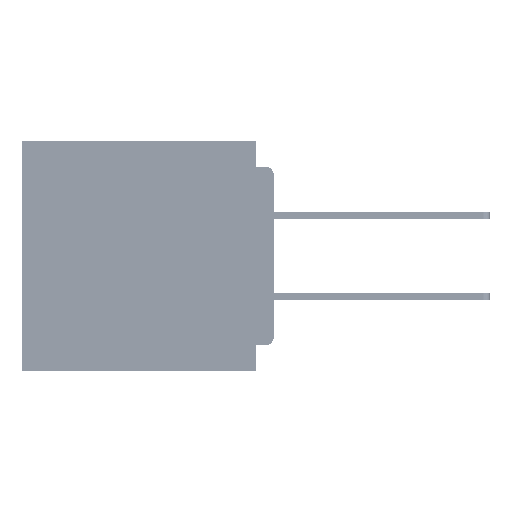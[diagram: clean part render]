
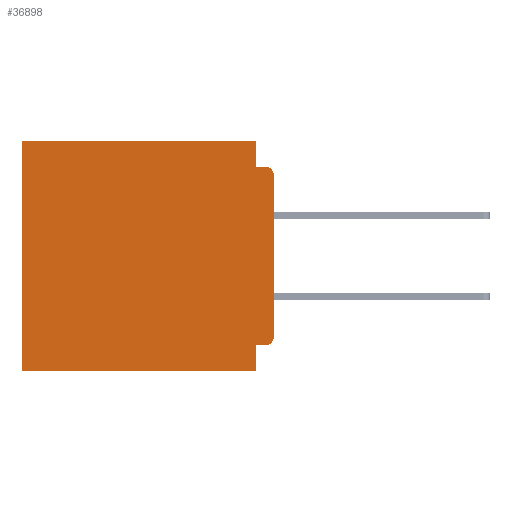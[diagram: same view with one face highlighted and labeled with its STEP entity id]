
A CAD part, left-side view. The second image highlights one B-rep face of the part: STEP entity #36898.
In plain terms, the highlighted planar face has unit normal (-1, 0, 0).
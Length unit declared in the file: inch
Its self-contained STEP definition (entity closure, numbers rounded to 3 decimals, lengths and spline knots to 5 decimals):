
#487 = VECTOR ( 'NONE', #36995, 39.37008 ) ;
#826 = DIRECTION ( 'NONE',  ( 0., -1., 0. ) ) ;
#1412 = EDGE_CURVE ( 'NONE', #47706, #27808, #40963, .T. ) ;
#2848 = DIRECTION ( 'NONE',  ( 0., 0., -1. ) ) ;
#3348 = ORIENTED_EDGE ( 'NONE', *, *, #37753, .F. ) ;
#4889 = VECTOR ( 'NONE', #64248, 39.37008 ) ;
#5545 = ORIENTED_EDGE ( 'NONE', *, *, #58320, .F. ) ;
#6227 = VECTOR ( 'NONE', #2848, 39.37008 ) ;
#6759 = CARTESIAN_POINT ( 'NONE',  ( 0.3, 0.031, -0.045 ) ) ;
#8298 = VERTEX_POINT ( 'NONE', #59583 ) ;
#8503 = LINE ( 'NONE', #52040, #49898 ) ;
#9433 = DIRECTION ( 'NONE',  ( 0., 0., -1. ) ) ;
#9648 = VECTOR ( 'NONE', #52516, 39.37008 ) ;
#11014 = EDGE_CURVE ( 'NONE', #61028, #56909, #8503, .T. ) ;
#11951 = CARTESIAN_POINT ( 'NONE',  ( 0.3, 0.015, -0.355 ) ) ;
#12437 = DIRECTION ( 'NONE',  ( 0., 0., -1. ) ) ;
#12934 = VERTEX_POINT ( 'NONE', #11951 ) ;
#19349 = CARTESIAN_POINT ( 'NONE',  ( 0.3, 0., -0.06 ) ) ;
#19749 = ORIENTED_EDGE ( 'NONE', *, *, #46625, .T. ) ;
#19824 = ORIENTED_EDGE ( 'NONE', *, *, #23410, .F. ) ;
#19858 = EDGE_CURVE ( 'NONE', #12934, #68266, #35274, .T. ) ;
#20147 = CARTESIAN_POINT ( 'NONE',  ( 0.3, 0., -0.4 ) ) ;
#20202 = DIRECTION ( 'NONE',  ( -1., 0., 0. ) ) ;
#20406 = DIRECTION ( 'NONE',  ( -1., 0., 0. ) ) ;
#21000 = EDGE_CURVE ( 'NONE', #47706, #51562, #29183, .T. ) ;
#22382 = LINE ( 'NONE', #28746, #41350 ) ;
#23410 = EDGE_CURVE ( 'NONE', #8298, #57819, #52736, .T. ) ;
#24838 = CARTESIAN_POINT ( 'NONE',  ( 0.3, 0.031, -0.4 ) ) ;
#25645 = CARTESIAN_POINT ( 'NONE',  ( 0.3, 0., -0.34 ) ) ;
#26329 = EDGE_CURVE ( 'NONE', #68266, #8298, #34617, .T. ) ;
#26506 = CARTESIAN_POINT ( 'NONE',  ( 0.3, 0., -0.355 ) ) ;
#27311 = ORIENTED_EDGE ( 'NONE', *, *, #19858, .F. ) ;
#27808 = VERTEX_POINT ( 'NONE', #51575 ) ;
#28276 = ORIENTED_EDGE ( 'NONE', *, *, #26329, .F. ) ;
#28746 = CARTESIAN_POINT ( 'NONE',  ( 0.3, 0.437, -0.4 ) ) ;
#29183 = LINE ( 'NONE', #58269, #487 ) ;
#30254 = DIRECTION ( 'NONE',  ( 0., 0., -1. ) ) ;
#30888 = PLANE ( 'NONE',  #50365 ) ;
#34617 = LINE ( 'NONE', #24838, #61672 ) ;
#35274 = LINE ( 'NONE', #26506, #4889 ) ;
#36310 = CARTESIAN_POINT ( 'NONE',  ( 0.3, 0., -0.4 ) ) ;
#36898 = ADVANCED_FACE ( 'NONE', ( #60589 ), #30888, .F. ) ;
#36995 = DIRECTION ( 'NONE',  ( 0., 0., -1. ) ) ;
#37696 = AXIS2_PLACEMENT_3D ( 'NONE', #52792, #20406, #58209 ) ;
#37753 = EDGE_CURVE ( 'NONE', #46304, #27808, #37769, .T. ) ;
#37769 = LINE ( 'NONE', #38598, #64764 ) ;
#38598 = CARTESIAN_POINT ( 'NONE',  ( 0.3, 0., -0.045 ) ) ;
#40812 = ORIENTED_EDGE ( 'NONE', *, *, #21000, .F. ) ;
#40963 = CIRCLE ( 'NONE', #52365, 0.015 ) ;
#41159 = ORIENTED_EDGE ( 'NONE', *, *, #1412, .T. ) ;
#41350 = VECTOR ( 'NONE', #12437, 39.37008 ) ;
#41779 = DIRECTION ( 'NONE',  ( 1., 0., 0. ) ) ;
#43084 = ORIENTED_EDGE ( 'NONE', *, *, #60879, .T. ) ;
#46196 = CARTESIAN_POINT ( 'NONE',  ( 0.3, 0.031, 0. ) ) ;
#46304 = VERTEX_POINT ( 'NONE', #6759 ) ;
#46625 = EDGE_CURVE ( 'NONE', #12934, #51562, #54628, .T. ) ;
#47706 = VERTEX_POINT ( 'NONE', #19349 ) ;
#49898 = VECTOR ( 'NONE', #57455, 39.37008 ) ;
#50365 = AXIS2_PLACEMENT_3D ( 'NONE', #36310, #41779, #9433 ) ;
#50807 = EDGE_LOOP ( 'NONE', ( #40812, #41159, #3348, #5545, #69065, #43084, #19824, #28276, #27311, #19749 ) ) ;
#51051 = LINE ( 'NONE', #56892, #6227 ) ;
#51562 = VERTEX_POINT ( 'NONE', #25645 ) ;
#51575 = CARTESIAN_POINT ( 'NONE',  ( 0.3, 0.015, -0.045 ) ) ;
#52040 = CARTESIAN_POINT ( 'NONE',  ( 0.3, 0., 0. ) ) ;
#52365 = AXIS2_PLACEMENT_3D ( 'NONE', #52585, #20202, #58007 ) ;
#52516 = DIRECTION ( 'NONE',  ( 0., 1., 0. ) ) ;
#52585 = CARTESIAN_POINT ( 'NONE',  ( 0.3, 0.015, -0.06 ) ) ;
#52736 = LINE ( 'NONE', #20147, #9648 ) ;
#52792 = CARTESIAN_POINT ( 'NONE',  ( 0.3, 0.015, -0.34 ) ) ;
#54628 = CIRCLE ( 'NONE', #37696, 0.015 ) ;
#54936 = CARTESIAN_POINT ( 'NONE',  ( 0.3, 0.437, 0. ) ) ;
#56892 = CARTESIAN_POINT ( 'NONE',  ( 0.3, 0.031, 0. ) ) ;
#56909 = VERTEX_POINT ( 'NONE', #54936 ) ;
#57455 = DIRECTION ( 'NONE',  ( 0., 1., 0. ) ) ;
#57819 = VERTEX_POINT ( 'NONE', #58160 ) ;
#58007 = DIRECTION ( 'NONE',  ( 0., 0., -1. ) ) ;
#58160 = CARTESIAN_POINT ( 'NONE',  ( 0.3, 0.437, -0.4 ) ) ;
#58209 = DIRECTION ( 'NONE',  ( 0., 0., -1. ) ) ;
#58269 = CARTESIAN_POINT ( 'NONE',  ( 0.3, 0., -0.4 ) ) ;
#58320 = EDGE_CURVE ( 'NONE', #61028, #46304, #51051, .T. ) ;
#59583 = CARTESIAN_POINT ( 'NONE',  ( 0.3, 0.031, -0.4 ) ) ;
#60589 = FACE_OUTER_BOUND ( 'NONE', #50807, .T. ) ;
#60879 = EDGE_CURVE ( 'NONE', #56909, #57819, #22382, .T. ) ;
#61028 = VERTEX_POINT ( 'NONE', #46196 ) ;
#61672 = VECTOR ( 'NONE', #30254, 39.37008 ) ;
#61834 = CARTESIAN_POINT ( 'NONE',  ( 0.3, 0.031, -0.355 ) ) ;
#64248 = DIRECTION ( 'NONE',  ( 0., 1., 0. ) ) ;
#64764 = VECTOR ( 'NONE', #826, 39.37008 ) ;
#68266 = VERTEX_POINT ( 'NONE', #61834 ) ;
#69065 = ORIENTED_EDGE ( 'NONE', *, *, #11014, .T. ) ;
